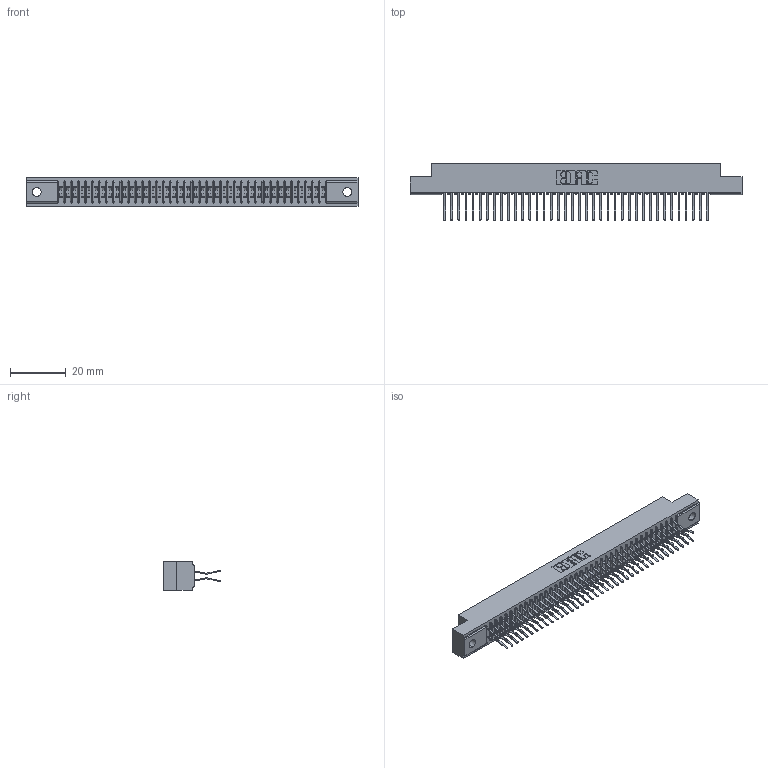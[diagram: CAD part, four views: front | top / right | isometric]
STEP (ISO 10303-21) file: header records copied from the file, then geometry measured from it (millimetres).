
FILE_DESCRIPTION (( 'STEP AP203' ), '1' );
FILE_NAME ('391-076-560-202.STEP', '2018-08-09T15:09:17', ( '' ), ( '' ), 'SwSTEP 2.0', 'SolidWorks 2016', '' );
FILE_SCHEMA (( 'CONFIG_CONTROL_DESIGN' ));
Length unit declared in the file: inch
Products named in the file (3): 391-076-560-202; 341 Part_.128 (3.25) Dia Mounting Holes; 341-292-001_341-292-160
Assembly tree (77 placements, depth 2):
  391-076-560-202
    341 Part_.128 (3.25) Dia Mounting Holes
    341-292-001_341-292-160  x76
Bounding box: 118.75 x 20.37 x 10.16 mm (x, y, z)
Volume: 8800.5 mm3; surface area: 15807.5 mm2
Topology: 77 solids, 77 shells, 5436 faces, 15782 edges, 10238 vertices
Faces by surface type: plane 3108, cylinder 2176, sphere 78, torus 74
Entity records: 46663 total; most frequent: CARTESIAN_POINT 7758, ORIENTED_EDGE 7708, DIRECTION 7536, EDGE_CURVE 3854, LINE 3104, VECTOR 3104, VERTEX_POINT 2438, AXIS2_PLACEMENT_3D 2216
